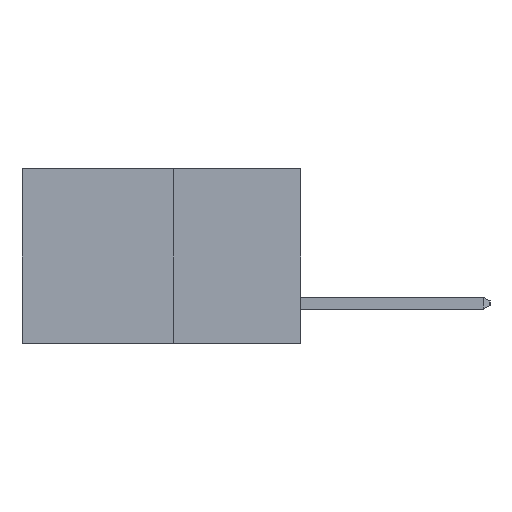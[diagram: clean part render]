
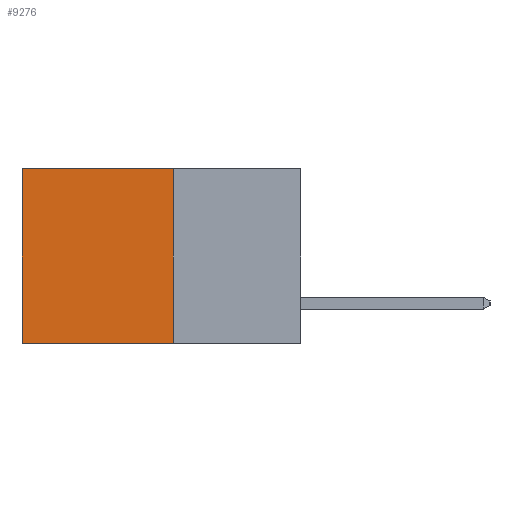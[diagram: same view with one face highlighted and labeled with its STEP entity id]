
A CAD part, left-side view. The second image highlights one B-rep face of the part: STEP entity #9276.
In plain terms, the highlighted planar face has unit normal (-1, 0, 0).
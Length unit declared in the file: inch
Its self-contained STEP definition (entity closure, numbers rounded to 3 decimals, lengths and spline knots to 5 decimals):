
#106 = CARTESIAN_POINT ( 'NONE',  ( 0.277, 0.27, 0. ) ) ;
#484 = ORIENTED_EDGE ( 'NONE', *, *, #8967, .T. ) ;
#539 = DIRECTION ( 'NONE',  ( 0., 0., -1. ) ) ;
#581 = DIRECTION ( 'NONE',  ( 1., 0., 0. ) ) ;
#664 = PLANE ( 'NONE',  #3366 ) ;
#671 = CARTESIAN_POINT ( 'NONE',  ( 0.277, 0.27, -0.37 ) ) ;
#1040 = CARTESIAN_POINT ( 'NONE',  ( 0.277, 0.59, 0. ) ) ;
#1080 = EDGE_CURVE ( 'NONE', #2740, #3889, #7702, .T. ) ;
#1237 = DIRECTION ( 'NONE',  ( 0., 0., -1. ) ) ;
#1335 = VECTOR ( 'NONE', #1237, 39.37008 ) ;
#1438 = CARTESIAN_POINT ( 'NONE',  ( 0.277, 0.59, -0.37 ) ) ;
#1590 = ORIENTED_EDGE ( 'NONE', *, *, #1080, .F. ) ;
#2332 = VECTOR ( 'NONE', #9316, 39.37008 ) ;
#2415 = EDGE_LOOP ( 'NONE', ( #2463, #2674, #1590, #484 ) ) ;
#2463 = ORIENTED_EDGE ( 'NONE', *, *, #9221, .T. ) ;
#2674 = ORIENTED_EDGE ( 'NONE', *, *, #8253, .F. ) ;
#2740 = VERTEX_POINT ( 'NONE', #106 ) ;
#3366 = AXIS2_PLACEMENT_3D ( 'NONE', #671, #581, #539 ) ;
#3440 = LINE ( 'NONE', #1438, #1335 ) ;
#3672 = VERTEX_POINT ( 'NONE', #9230 ) ;
#3889 = VERTEX_POINT ( 'NONE', #5819 ) ;
#3985 = DIRECTION ( 'NONE',  ( 0., 1., 0. ) ) ;
#4011 = CARTESIAN_POINT ( 'NONE',  ( 0.277, 0.27, 0. ) ) ;
#4277 = CARTESIAN_POINT ( 'NONE',  ( 0.277, 0.27, -0.37 ) ) ;
#5819 = CARTESIAN_POINT ( 'NONE',  ( 0.277, 0.27, -0.37 ) ) ;
#6371 = VERTEX_POINT ( 'NONE', #1040 ) ;
#6380 = VECTOR ( 'NONE', #8567, 39.37008 ) ;
#7082 = FACE_OUTER_BOUND ( 'NONE', #2415, .T. ) ;
#7191 = VECTOR ( 'NONE', #3985, 39.37008 ) ;
#7403 = LINE ( 'NONE', #4011, #7191 ) ;
#7702 = LINE ( 'NONE', #4277, #2332 ) ;
#8253 = EDGE_CURVE ( 'NONE', #3889, #3672, #8404, .T. ) ;
#8404 = LINE ( 'NONE', #8664, #6380 ) ;
#8567 = DIRECTION ( 'NONE',  ( 0., 1., 0. ) ) ;
#8664 = CARTESIAN_POINT ( 'NONE',  ( 0.277, 0.27, -0.37 ) ) ;
#8967 = EDGE_CURVE ( 'NONE', #2740, #6371, #7403, .T. ) ;
#9221 = EDGE_CURVE ( 'NONE', #6371, #3672, #3440, .T. ) ;
#9230 = CARTESIAN_POINT ( 'NONE',  ( 0.277, 0.59, -0.37 ) ) ;
#9276 = ADVANCED_FACE ( 'NONE', ( #7082 ), #664, .F. ) ;
#9316 = DIRECTION ( 'NONE',  ( 0., 0., -1. ) ) ;
